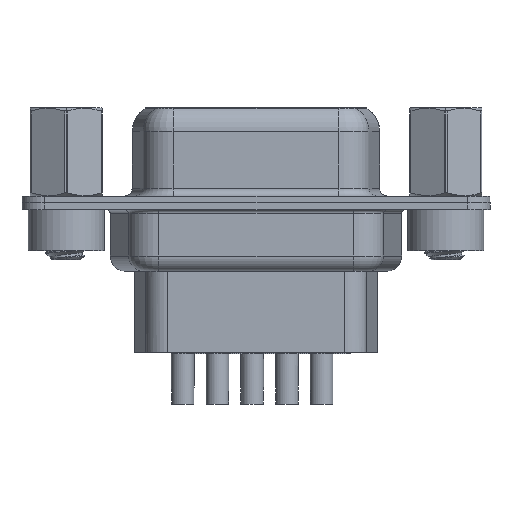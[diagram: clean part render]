
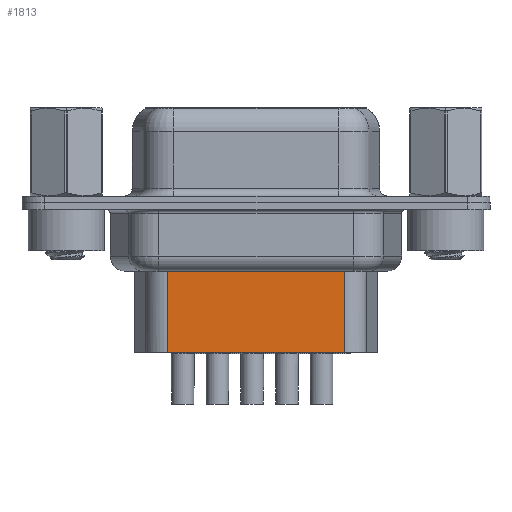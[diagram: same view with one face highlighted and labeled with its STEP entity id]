
A CAD part, front view. The second image highlights one B-rep face of the part: STEP entity #1813.
In plain terms, the highlighted planar face has unit normal (0, -1, 0).
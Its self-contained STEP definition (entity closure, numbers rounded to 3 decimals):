
#264 = VECTOR ( 'NONE', #25292, 1000. ) ;
#330 = CARTESIAN_POINT ( 'NONE',  ( 6.701, -3.5, -9.85 ) ) ;
#1813 = ADVANCED_FACE ( 'NONE', ( #29153 ), #8460, .T. ) ;
#2615 = VECTOR ( 'NONE', #19388, 1000. ) ;
#4920 = CARTESIAN_POINT ( 'NONE',  ( 18.289, -3.5, -3.1 ) ) ;
#6648 = ORIENTED_EDGE ( 'NONE', *, *, #9630, .F. ) ;
#6797 = VERTEX_POINT ( 'NONE', #28238 ) ;
#6983 = LINE ( 'NONE', #330, #264 ) ;
#7545 = LINE ( 'NONE', #10066, #12900 ) ;
#8460 = PLANE ( 'NONE',  #26060 ) ;
#8608 = LINE ( 'NONE', #10170, #2615 ) ;
#9616 = CARTESIAN_POINT ( 'NONE',  ( 18.289, -3.5, -4.097 ) ) ;
#9630 = EDGE_CURVE ( 'NONE', #6797, #19180, #6983, .T. ) ;
#9692 = LINE ( 'NONE', #4920, #21142 ) ;
#9969 = ORIENTED_EDGE ( 'NONE', *, *, #16562, .T. ) ;
#10066 = CARTESIAN_POINT ( 'NONE',  ( 6.701, -3.5, -3.1 ) ) ;
#10170 = CARTESIAN_POINT ( 'NONE',  ( 6.454, -3.5, -4.097 ) ) ;
#11500 = EDGE_LOOP ( 'NONE', ( #17090, #9969, #26320, #6648 ) ) ;
#12387 = DIRECTION ( 'NONE',  ( 0., 0., -1. ) ) ;
#12900 = VECTOR ( 'NONE', #12387, 1000. ) ;
#14356 = VERTEX_POINT ( 'NONE', #9616 ) ;
#14984 = DIRECTION ( 'NONE',  ( 0., -1., 0. ) ) ;
#15146 = EDGE_CURVE ( 'NONE', #14356, #6797, #9692, .T. ) ;
#15551 = CARTESIAN_POINT ( 'NONE',  ( 6.701, -3.5, -3.1 ) ) ;
#15677 = VERTEX_POINT ( 'NONE', #17956 ) ;
#16562 = EDGE_CURVE ( 'NONE', #14356, #15677, #8608, .T. ) ;
#17090 = ORIENTED_EDGE ( 'NONE', *, *, #15146, .F. ) ;
#17956 = CARTESIAN_POINT ( 'NONE',  ( 6.701, -3.5, -4.097 ) ) ;
#19180 = VERTEX_POINT ( 'NONE', #24250 ) ;
#19388 = DIRECTION ( 'NONE',  ( -1., 0., 0. ) ) ;
#20118 = DIRECTION ( 'NONE',  ( 1., 0., 0. ) ) ;
#21142 = VECTOR ( 'NONE', #27712, 1000. ) ;
#24250 = CARTESIAN_POINT ( 'NONE',  ( 6.701, -3.5, -9.85 ) ) ;
#25221 = EDGE_CURVE ( 'NONE', #15677, #19180, #7545, .T. ) ;
#25292 = DIRECTION ( 'NONE',  ( -1., 0., 0. ) ) ;
#26060 = AXIS2_PLACEMENT_3D ( 'NONE', #15551, #14984, #20118 ) ;
#26320 = ORIENTED_EDGE ( 'NONE', *, *, #25221, .T. ) ;
#27712 = DIRECTION ( 'NONE',  ( 0., 0., -1. ) ) ;
#28238 = CARTESIAN_POINT ( 'NONE',  ( 18.289, -3.5, -9.85 ) ) ;
#29153 = FACE_OUTER_BOUND ( 'NONE', #11500, .T. ) ;
